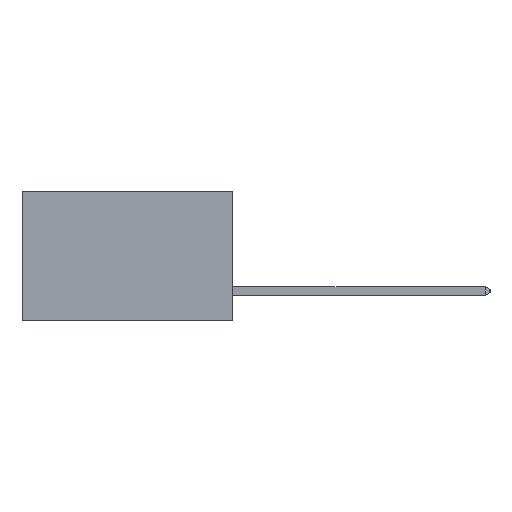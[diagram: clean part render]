
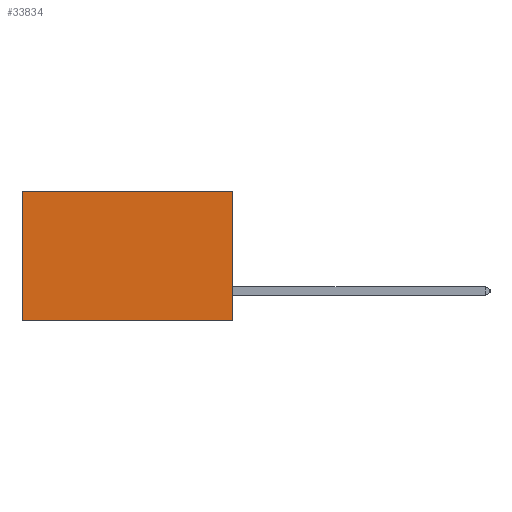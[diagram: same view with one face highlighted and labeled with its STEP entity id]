
A CAD part, left-side view. The second image highlights one B-rep face of the part: STEP entity #33834.
In plain terms, the highlighted planar face has unit normal (-1, 0, 0).
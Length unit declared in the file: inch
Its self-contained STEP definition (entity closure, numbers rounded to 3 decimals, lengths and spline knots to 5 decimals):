
#662 = CARTESIAN_POINT ( 'NONE',  ( 0.2875, 0., 0. ) ) ;
#1160 = VERTEX_POINT ( 'NONE', #2029 ) ;
#2029 = CARTESIAN_POINT ( 'NONE',  ( 0.2875, 0., -0.37 ) ) ;
#4321 = CARTESIAN_POINT ( 'NONE',  ( 0.2875, 0., 0. ) ) ;
#4587 = LINE ( 'NONE', #9236, #25316 ) ;
#4844 = ORIENTED_EDGE ( 'NONE', *, *, #16778, .T. ) ;
#5408 = EDGE_LOOP ( 'NONE', ( #27984, #23877, #7294, #4844 ) ) ;
#5496 = AXIS2_PLACEMENT_3D ( 'NONE', #4321, #24932, #7295 ) ;
#6762 = LINE ( 'NONE', #33546, #36848 ) ;
#6793 = FACE_OUTER_BOUND ( 'NONE', #5408, .T. ) ;
#7294 = ORIENTED_EDGE ( 'NONE', *, *, #23936, .F. ) ;
#7295 = DIRECTION ( 'NONE',  ( 0., 0., -1. ) ) ;
#9236 = CARTESIAN_POINT ( 'NONE',  ( 0.2875, 0., -0.37 ) ) ;
#9511 = DIRECTION ( 'NONE',  ( 0., 1., 0. ) ) ;
#11862 = VERTEX_POINT ( 'NONE', #28631 ) ;
#12104 = VECTOR ( 'NONE', #37712, 39.37008 ) ;
#12227 = DIRECTION ( 'NONE',  ( 0., 1., 0. ) ) ;
#16778 = EDGE_CURVE ( 'NONE', #27853, #23029, #24208, .T. ) ;
#17612 = CARTESIAN_POINT ( 'NONE',  ( 0.2875, 0.6, 0. ) ) ;
#19094 = PLANE ( 'NONE',  #5496 ) ;
#20464 = CARTESIAN_POINT ( 'NONE',  ( 0.2875, 0.6, 0. ) ) ;
#23029 = VERTEX_POINT ( 'NONE', #17612 ) ;
#23877 = ORIENTED_EDGE ( 'NONE', *, *, #24375, .F. ) ;
#23936 = EDGE_CURVE ( 'NONE', #27853, #1160, #6762, .T. ) ;
#24208 = LINE ( 'NONE', #662, #29997 ) ;
#24375 = EDGE_CURVE ( 'NONE', #1160, #11862, #4587, .T. ) ;
#24932 = DIRECTION ( 'NONE',  ( 1., 0., 0. ) ) ;
#25316 = VECTOR ( 'NONE', #12227, 39.37008 ) ;
#27853 = VERTEX_POINT ( 'NONE', #29473 ) ;
#27973 = DIRECTION ( 'NONE',  ( 0., 0., -1. ) ) ;
#27984 = ORIENTED_EDGE ( 'NONE', *, *, #31415, .T. ) ;
#28631 = CARTESIAN_POINT ( 'NONE',  ( 0.2875, 0.6, -0.37 ) ) ;
#29473 = CARTESIAN_POINT ( 'NONE',  ( 0.2875, 0., 0. ) ) ;
#29997 = VECTOR ( 'NONE', #9511, 39.37008 ) ;
#31415 = EDGE_CURVE ( 'NONE', #23029, #11862, #34325, .T. ) ;
#33546 = CARTESIAN_POINT ( 'NONE',  ( 0.2875, 0., 0. ) ) ;
#33834 = ADVANCED_FACE ( 'NONE', ( #6793 ), #19094, .F. ) ;
#34325 = LINE ( 'NONE', #20464, #12104 ) ;
#36848 = VECTOR ( 'NONE', #27973, 39.37008 ) ;
#37712 = DIRECTION ( 'NONE',  ( 0., 0., -1. ) ) ;
